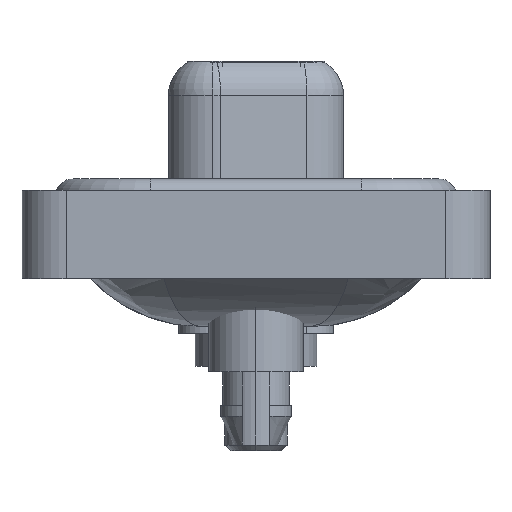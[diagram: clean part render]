
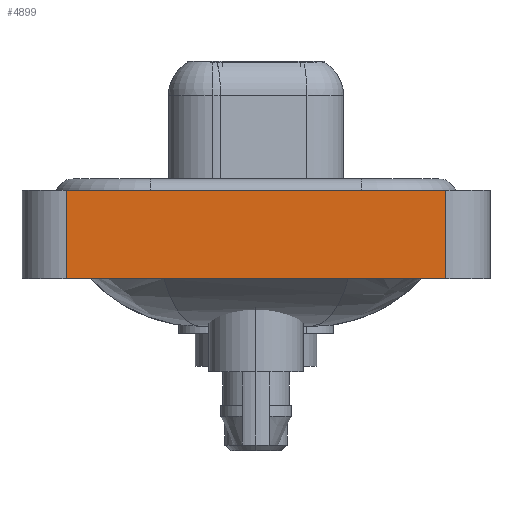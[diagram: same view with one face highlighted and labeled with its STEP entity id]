
A CAD part, left-side view. The second image highlights one B-rep face of the part: STEP entity #4899.
In plain terms, the highlighted planar face has unit normal (-1, 0, 0).
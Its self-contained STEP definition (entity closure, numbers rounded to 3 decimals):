
#70 = CARTESIAN_POINT ( 'NONE',  ( -7.35, -8.55, 0.4 ) ) ;
#106 = EDGE_CURVE ( 'NONE', #13843, #2723, #15176, .T. ) ;
#554 = DIRECTION ( 'NONE',  ( 0., 0., 1. ) ) ;
#588 = VECTOR ( 'NONE', #554, 1000. ) ;
#2674 = CARTESIAN_POINT ( 'NONE',  ( -7.35, -8.55, -3.6 ) ) ;
#2723 = VERTEX_POINT ( 'NONE', #70 ) ;
#3868 = CARTESIAN_POINT ( 'NONE',  ( -7.35, 8.55, -3.6 ) ) ;
#4042 = CARTESIAN_POINT ( 'NONE',  ( -7.35, 8.55, 0.4 ) ) ;
#4215 = LINE ( 'NONE', #2674, #9552 ) ;
#4594 = VERTEX_POINT ( 'NONE', #3868 ) ;
#4899 = ADVANCED_FACE ( 'NONE', ( #8165 ), #17747, .T. ) ;
#5360 = EDGE_LOOP ( 'NONE', ( #9883, #8650, #13270, #6509 ) ) ;
#6509 = ORIENTED_EDGE ( 'NONE', *, *, #8578, .T. ) ;
#7315 = VERTEX_POINT ( 'NONE', #15197 ) ;
#7719 = VECTOR ( 'NONE', #11110, 1000. ) ;
#8077 = DIRECTION ( 'NONE',  ( 0., 0., 1. ) ) ;
#8165 = FACE_OUTER_BOUND ( 'NONE', #5360, .T. ) ;
#8472 = LINE ( 'NONE', #11204, #7719 ) ;
#8578 = EDGE_CURVE ( 'NONE', #4594, #7315, #8472, .T. ) ;
#8650 = ORIENTED_EDGE ( 'NONE', *, *, #106, .F. ) ;
#8809 = VECTOR ( 'NONE', #13703, 1000. ) ;
#9400 = AXIS2_PLACEMENT_3D ( 'NONE', #9797, #16554, #8077 ) ;
#9552 = VECTOR ( 'NONE', #17910, 1000. ) ;
#9797 = CARTESIAN_POINT ( 'NONE',  ( -7.35, -8.55, -3.6 ) ) ;
#9883 = ORIENTED_EDGE ( 'NONE', *, *, #12309, .T. ) ;
#10305 = LINE ( 'NONE', #13029, #588 ) ;
#11110 = DIRECTION ( 'NONE',  ( 0., -1., 0. ) ) ;
#11204 = CARTESIAN_POINT ( 'NONE',  ( -7.35, -8.55, -3.6 ) ) ;
#12309 = EDGE_CURVE ( 'NONE', #7315, #2723, #4215, .T. ) ;
#13029 = CARTESIAN_POINT ( 'NONE',  ( -7.35, 8.55, -3.6 ) ) ;
#13270 = ORIENTED_EDGE ( 'NONE', *, *, #14522, .F. ) ;
#13703 = DIRECTION ( 'NONE',  ( 0., -1., 0. ) ) ;
#13843 = VERTEX_POINT ( 'NONE', #4042 ) ;
#13887 = CARTESIAN_POINT ( 'NONE',  ( -7.35, -8.55, 0.4 ) ) ;
#14522 = EDGE_CURVE ( 'NONE', #4594, #13843, #10305, .T. ) ;
#15176 = LINE ( 'NONE', #13887, #8809 ) ;
#15197 = CARTESIAN_POINT ( 'NONE',  ( -7.35, -8.55, -3.6 ) ) ;
#16554 = DIRECTION ( 'NONE',  ( -1., 0., 0. ) ) ;
#17747 = PLANE ( 'NONE',  #9400 ) ;
#17910 = DIRECTION ( 'NONE',  ( 0., 0., 1. ) ) ;
